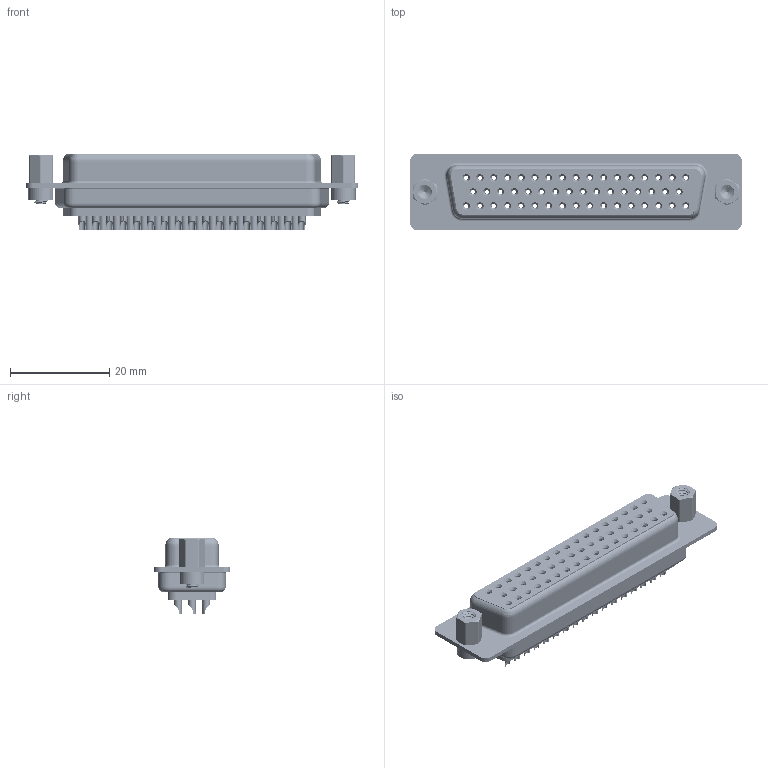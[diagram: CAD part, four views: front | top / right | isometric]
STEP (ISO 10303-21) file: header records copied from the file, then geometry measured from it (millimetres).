
FILE_DESCRIPTION (( 'STEP AP203' ), '1' );
FILE_NAME ('628-050-622-043.STEP', '2021-04-22T20:49:33', ( '' ), ( '' ), 'SwSTEP 2.0', 'SolidWorks 2020', '' );
FILE_SCHEMA (( 'CONFIG_CONTROL_DESIGN' ));
Length unit declared in the file: millimetre
Products named in the file (9): 628 Contact Row 3_22L; 628 4-40 Threaded Rivet; 628 Housing_50 LP; 628 Contact Row 1_22L; 628 Shell Front_50 Contacts; 628 Shell Rear_50 Contacts; 628-050-622-043; 628 Contact Row 2_22M; 628 4-40 Hex Standoff
Assembly tree (57 placements, depth 2):
  628-050-622-043
    628 Housing_50 LP
    628 Shell Front_50 Contacts
    628 Shell Rear_50 Contacts
    628 Contact Row 1_22L  x17
    628 Contact Row 2_22M  x16
    628 Contact Row 3_22L  x17
    628 4-40 Threaded Rivet  x2
    628 4-40 Hex Standoff  x2
Bounding box: 67 x 15.4 x 15.5 mm (x, y, z)
Volume: 6976 mm3; surface area: 16085.4 mm2
Topology: 57 solids, 57 shells, 4851 faces, 12319 edges, 7743 vertices
Faces by surface type: cylinder 1457, plane 1139, bspline 1018, torus 957, cone 280
Entity records: 42758 total; most frequent: CARTESIAN_POINT 12827, DIRECTION 6128, ORIENTED_EDGE 5526, EDGE_CURVE 2763, AXIS2_PLACEMENT_3D 2584, VERTEX_POINT 1755, EDGE_LOOP 1460, CIRCLE 1408
